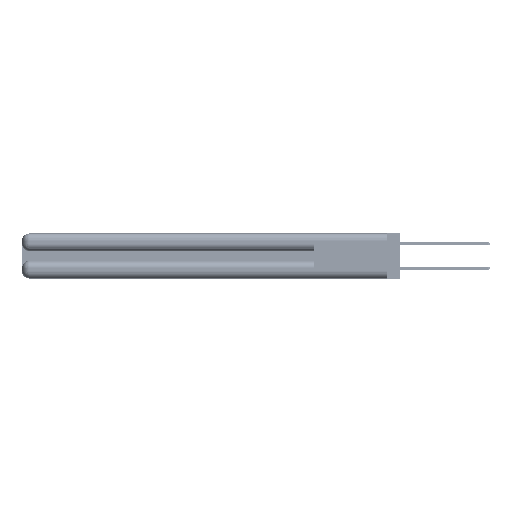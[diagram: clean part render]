
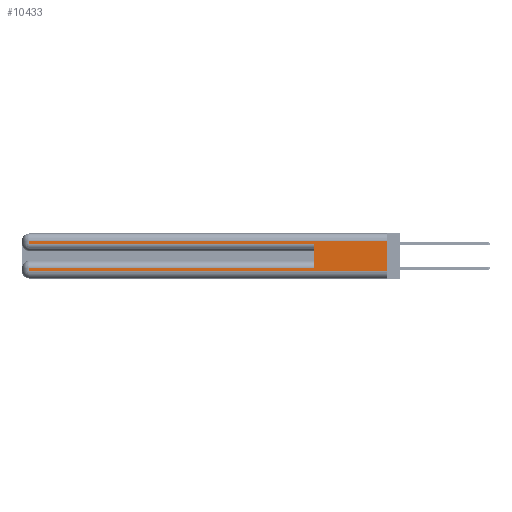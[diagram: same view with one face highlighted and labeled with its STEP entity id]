
A CAD part, left-side view. The second image highlights one B-rep face of the part: STEP entity #10433.
In plain terms, the highlighted planar face has unit normal (-1, 0, 0).
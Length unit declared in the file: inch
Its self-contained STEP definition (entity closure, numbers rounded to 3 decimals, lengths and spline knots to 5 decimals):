
#278 = EDGE_CURVE ( 'NONE', #33504, #46766, #2558, .T. ) ;
#1654 = DIRECTION ( 'NONE',  ( 0., 0., 1. ) ) ;
#2423 = ORIENTED_EDGE ( 'NONE', *, *, #9800, .T. ) ;
#2558 = LINE ( 'NONE', #39388, #22618 ) ;
#2923 = CARTESIAN_POINT ( 'NONE',  ( 0., 2.94, 0.37 ) ) ;
#2936 = EDGE_CURVE ( 'NONE', #20969, #42794, #43618, .T. ) ;
#4868 = LINE ( 'NONE', #2923, #35652 ) ;
#4947 = ORIENTED_EDGE ( 'NONE', *, *, #43942, .T. ) ;
#5526 = CARTESIAN_POINT ( 'NONE',  ( 0., 0., 0.37 ) ) ;
#5923 = EDGE_CURVE ( 'NONE', #46766, #42794, #31907, .T. ) ;
#8366 = CARTESIAN_POINT ( 'NONE',  ( 0., 0., 0.06 ) ) ;
#9530 = ORIENTED_EDGE ( 'NONE', *, *, #278, .T. ) ;
#9738 = PLANE ( 'NONE',  #24930 ) ;
#9800 = EDGE_CURVE ( 'NONE', #46981, #42530, #13773, .T. ) ;
#10433 = ADVANCED_FACE ( 'NONE', ( #40077 ), #9738, .F. ) ;
#10526 = ORIENTED_EDGE ( 'NONE', *, *, #2936, .F. ) ;
#10957 = DIRECTION ( 'NONE',  ( 0., 0., -1. ) ) ;
#11530 = CARTESIAN_POINT ( 'NONE',  ( 0., 0., 0.06 ) ) ;
#11970 = CARTESIAN_POINT ( 'NONE',  ( 0., 0., 0.31 ) ) ;
#13210 = CARTESIAN_POINT ( 'NONE',  ( 0., 0.6, 0.145 ) ) ;
#13773 = LINE ( 'NONE', #16399, #49594 ) ;
#14434 = VERTEX_POINT ( 'NONE', #23872 ) ;
#14690 = CARTESIAN_POINT ( 'NONE',  ( 0., 2.94, 0.06 ) ) ;
#15808 = DIRECTION ( 'NONE',  ( 0., 1., 0. ) ) ;
#16399 = CARTESIAN_POINT ( 'NONE',  ( 0., 0., 0.285 ) ) ;
#17818 = CARTESIAN_POINT ( 'NONE',  ( 0., 0., 0.31 ) ) ;
#19434 = EDGE_CURVE ( 'NONE', #14434, #33504, #25396, .T. ) ;
#19976 = VECTOR ( 'NONE', #1654, 39.37008 ) ;
#20969 = VERTEX_POINT ( 'NONE', #17818 ) ;
#22295 = CARTESIAN_POINT ( 'NONE',  ( 0., 0., 0.085 ) ) ;
#22618 = VECTOR ( 'NONE', #10957, 39.37008 ) ;
#23506 = VECTOR ( 'NONE', #51439, 39.37008 ) ;
#23872 = CARTESIAN_POINT ( 'NONE',  ( 0., 0.6, 0.085 ) ) ;
#24930 = AXIS2_PLACEMENT_3D ( 'NONE', #5526, #49913, #33264 ) ;
#25396 = LINE ( 'NONE', #22295, #23506 ) ;
#27668 = CARTESIAN_POINT ( 'NONE',  ( 0., 2.94, 0.285 ) ) ;
#28526 = VECTOR ( 'NONE', #15808, 39.37008 ) ;
#28685 = DIRECTION ( 'NONE',  ( 0., -1., 0. ) ) ;
#29169 = DIRECTION ( 'NONE',  ( 0., 0., -1. ) ) ;
#29811 = ORIENTED_EDGE ( 'NONE', *, *, #5923, .T. ) ;
#30462 = DIRECTION ( 'NONE',  ( 0., 0., -1. ) ) ;
#31907 = LINE ( 'NONE', #11530, #35715 ) ;
#33098 = ORIENTED_EDGE ( 'NONE', *, *, #19434, .T. ) ;
#33264 = DIRECTION ( 'NONE',  ( 0., 0., -1. ) ) ;
#33504 = VERTEX_POINT ( 'NONE', #44139 ) ;
#34046 = CARTESIAN_POINT ( 'NONE',  ( 0., 0.6, 0.285 ) ) ;
#35652 = VECTOR ( 'NONE', #30462, 39.37008 ) ;
#35708 = ORIENTED_EDGE ( 'NONE', *, *, #38474, .F. ) ;
#35715 = VECTOR ( 'NONE', #39614, 39.37008 ) ;
#37210 = EDGE_LOOP ( 'NONE', ( #10526, #4947, #41926, #2423, #35708, #33098, #9530, #29811 ) ) ;
#37297 = CARTESIAN_POINT ( 'NONE',  ( 0., 0., 0.37 ) ) ;
#38474 = EDGE_CURVE ( 'NONE', #14434, #42530, #45781, .T. ) ;
#39333 = VERTEX_POINT ( 'NONE', #42816 ) ;
#39388 = CARTESIAN_POINT ( 'NONE',  ( 0., 2.94, 0.37 ) ) ;
#39614 = DIRECTION ( 'NONE',  ( 0., -1., 0. ) ) ;
#40077 = FACE_OUTER_BOUND ( 'NONE', #37210, .T. ) ;
#40464 = VECTOR ( 'NONE', #29169, 39.37008 ) ;
#41926 = ORIENTED_EDGE ( 'NONE', *, *, #50133, .T. ) ;
#42530 = VERTEX_POINT ( 'NONE', #34046 ) ;
#42794 = VERTEX_POINT ( 'NONE', #8366 ) ;
#42816 = CARTESIAN_POINT ( 'NONE',  ( 0., 2.94, 0.31 ) ) ;
#43618 = LINE ( 'NONE', #37297, #40464 ) ;
#43942 = EDGE_CURVE ( 'NONE', #20969, #39333, #51150, .T. ) ;
#44139 = CARTESIAN_POINT ( 'NONE',  ( 0., 2.94, 0.085 ) ) ;
#45781 = LINE ( 'NONE', #13210, #19976 ) ;
#46766 = VERTEX_POINT ( 'NONE', #14690 ) ;
#46981 = VERTEX_POINT ( 'NONE', #27668 ) ;
#49594 = VECTOR ( 'NONE', #28685, 39.37008 ) ;
#49913 = DIRECTION ( 'NONE',  ( 1., 0., 0. ) ) ;
#50133 = EDGE_CURVE ( 'NONE', #39333, #46981, #4868, .T. ) ;
#51150 = LINE ( 'NONE', #11970, #28526 ) ;
#51439 = DIRECTION ( 'NONE',  ( 0., 1., 0. ) ) ;
